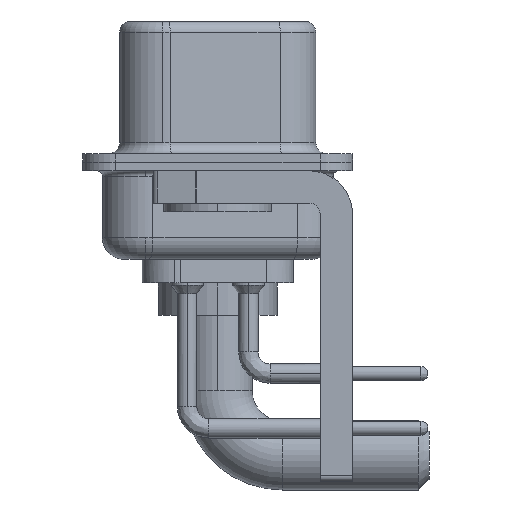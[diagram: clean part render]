
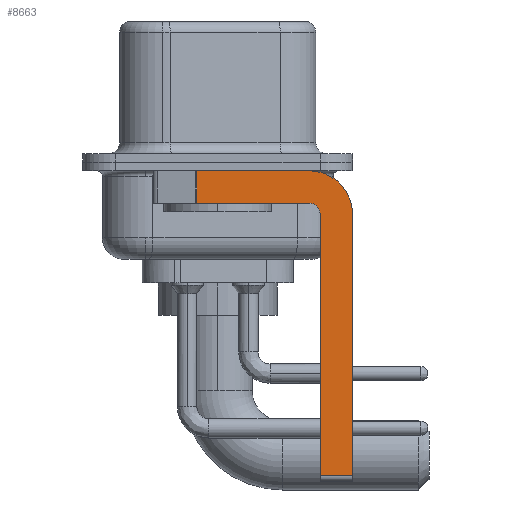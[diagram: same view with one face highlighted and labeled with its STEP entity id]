
A CAD part, left-side view. The second image highlights one B-rep face of the part: STEP entity #8663.
In plain terms, the highlighted planar face has unit normal (-1, 0, 0).
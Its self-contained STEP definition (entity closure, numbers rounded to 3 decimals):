
#326 = LINE ( 'NONE', #4904, #14299 ) ;
#381 = EDGE_LOOP ( 'NONE', ( #6451, #1122, #2265, #10198, #14067, #3243, #6836, #4642 ) ) ;
#592 = EDGE_CURVE ( 'NONE', #9281, #4453, #15542, .T. ) ;
#1122 = ORIENTED_EDGE ( 'NONE', *, *, #16740, .T. ) ;
#1453 = CARTESIAN_POINT ( 'NONE',  ( -2.9, -4.25, -14.55 ) ) ;
#1606 = CARTESIAN_POINT ( 'NONE',  ( -2.9, 0.978, -1.9 ) ) ;
#1762 = DIRECTION ( 'NONE',  ( 1., 0., 0. ) ) ;
#2265 = ORIENTED_EDGE ( 'NONE', *, *, #8522, .F. ) ;
#2855 = CARTESIAN_POINT ( 'NONE',  ( -2.9, -6.25, -2.4 ) ) ;
#2941 = CARTESIAN_POINT ( 'NONE',  ( -2.9, -4.25, -2.4 ) ) ;
#3243 = ORIENTED_EDGE ( 'NONE', *, *, #9214, .T. ) ;
#3575 = CARTESIAN_POINT ( 'NONE',  ( -2.9, -6.25, -14.55 ) ) ;
#4165 = CARTESIAN_POINT ( 'NONE',  ( -2.9, -4.25, -2.4 ) ) ;
#4379 = PLANE ( 'NONE',  #12776 ) ;
#4453 = VERTEX_POINT ( 'NONE', #3575 ) ;
#4535 = CARTESIAN_POINT ( 'NONE',  ( -2.9, -4.75, -14.55 ) ) ;
#4642 = ORIENTED_EDGE ( 'NONE', *, *, #9434, .F. ) ;
#4767 = CARTESIAN_POINT ( 'NONE',  ( -2.9, 3., -0.4 ) ) ;
#4777 = CARTESIAN_POINT ( 'NONE',  ( -2.9, -4.25, -1.9 ) ) ;
#4795 = CARTESIAN_POINT ( 'NONE',  ( -2.9, -4.25, -2.4 ) ) ;
#4904 = CARTESIAN_POINT ( 'NONE',  ( -2.9, -4.75, -14.8 ) ) ;
#5176 = CARTESIAN_POINT ( 'NONE',  ( -2.9, 0.978, -1.9 ) ) ;
#5312 = VECTOR ( 'NONE', #15082, 1000. ) ;
#5384 = VERTEX_POINT ( 'NONE', #14623 ) ;
#5407 = VECTOR ( 'NONE', #12711, 1000. ) ;
#6291 = AXIS2_PLACEMENT_3D ( 'NONE', #4795, #1762, #14062 ) ;
#6440 = EDGE_CURVE ( 'NONE', #13763, #9054, #326, .T. ) ;
#6451 = ORIENTED_EDGE ( 'NONE', *, *, #14649, .F. ) ;
#6836 = ORIENTED_EDGE ( 'NONE', *, *, #592, .F. ) ;
#7570 = VECTOR ( 'NONE', #18200, 1000. ) ;
#7827 = CARTESIAN_POINT ( 'NONE',  ( -2.9, -6.25, -2.4 ) ) ;
#7907 = VERTEX_POINT ( 'NONE', #15812 ) ;
#8522 = EDGE_CURVE ( 'NONE', #17961, #13775, #12016, .T. ) ;
#8663 = ADVANCED_FACE ( 'NONE', ( #19833 ), #4379, .F. ) ;
#9054 = VERTEX_POINT ( 'NONE', #15979 ) ;
#9214 = EDGE_CURVE ( 'NONE', #13763, #4453, #16697, .T. ) ;
#9272 = LINE ( 'NONE', #4767, #15971 ) ;
#9281 = VERTEX_POINT ( 'NONE', #2855 ) ;
#9434 = EDGE_CURVE ( 'NONE', #7907, #9281, #12466, .T. ) ;
#9878 = LINE ( 'NONE', #5176, #15202 ) ;
#10198 = ORIENTED_EDGE ( 'NONE', *, *, #12774, .F. ) ;
#10498 = CARTESIAN_POINT ( 'NONE',  ( -2.9, -4.25, -1.9 ) ) ;
#10582 = DIRECTION ( 'NONE',  ( -1., 0., 0. ) ) ;
#10595 = DIRECTION ( 'NONE',  ( 1., 0., 0. ) ) ;
#11135 = DIRECTION ( 'NONE',  ( 0., 0., 1. ) ) ;
#12016 = LINE ( 'NONE', #10498, #7570 ) ;
#12466 = CIRCLE ( 'NONE', #6291, 2. ) ;
#12711 = DIRECTION ( 'NONE',  ( 0., 0., -1. ) ) ;
#12774 = EDGE_CURVE ( 'NONE', #9054, #17961, #13972, .T. ) ;
#12776 = AXIS2_PLACEMENT_3D ( 'NONE', #2941, #10595, #16778 ) ;
#13763 = VERTEX_POINT ( 'NONE', #4535 ) ;
#13775 = VERTEX_POINT ( 'NONE', #1606 ) ;
#13972 = CIRCLE ( 'NONE', #14625, 0.5 ) ;
#14062 = DIRECTION ( 'NONE',  ( 0., 0., -1. ) ) ;
#14067 = ORIENTED_EDGE ( 'NONE', *, *, #6440, .F. ) ;
#14299 = VECTOR ( 'NONE', #11135, 1000. ) ;
#14437 = DIRECTION ( 'NONE',  ( 0., 0., -1. ) ) ;
#14623 = CARTESIAN_POINT ( 'NONE',  ( -2.9, 0.978, -0.4 ) ) ;
#14625 = AXIS2_PLACEMENT_3D ( 'NONE', #4165, #10582, #18083 ) ;
#14649 = EDGE_CURVE ( 'NONE', #5384, #7907, #9272, .T. ) ;
#15082 = DIRECTION ( 'NONE',  ( 0., -1., 0. ) ) ;
#15202 = VECTOR ( 'NONE', #14437, 1000. ) ;
#15542 = LINE ( 'NONE', #7827, #5407 ) ;
#15812 = CARTESIAN_POINT ( 'NONE',  ( -2.9, -4.25, -0.4 ) ) ;
#15971 = VECTOR ( 'NONE', #18795, 1000. ) ;
#15979 = CARTESIAN_POINT ( 'NONE',  ( -2.9, -4.75, -2.4 ) ) ;
#16697 = LINE ( 'NONE', #1453, #5312 ) ;
#16740 = EDGE_CURVE ( 'NONE', #5384, #13775, #9878, .T. ) ;
#16778 = DIRECTION ( 'NONE',  ( 0., 0., -1. ) ) ;
#17961 = VERTEX_POINT ( 'NONE', #4777 ) ;
#18083 = DIRECTION ( 'NONE',  ( 0., 0., 1. ) ) ;
#18200 = DIRECTION ( 'NONE',  ( 0., 1., 0. ) ) ;
#18795 = DIRECTION ( 'NONE',  ( 0., -1., 0. ) ) ;
#19833 = FACE_OUTER_BOUND ( 'NONE', #381, .T. ) ;
